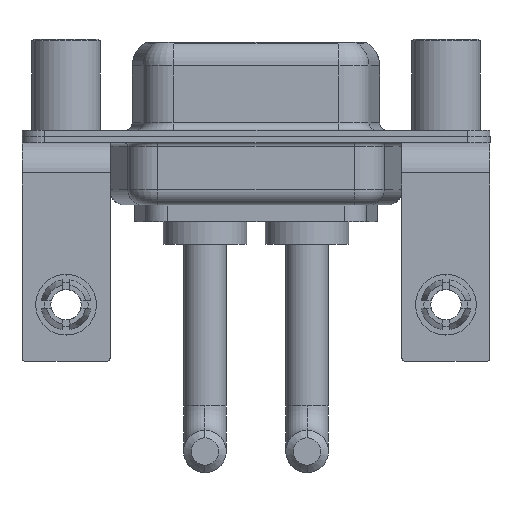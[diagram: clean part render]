
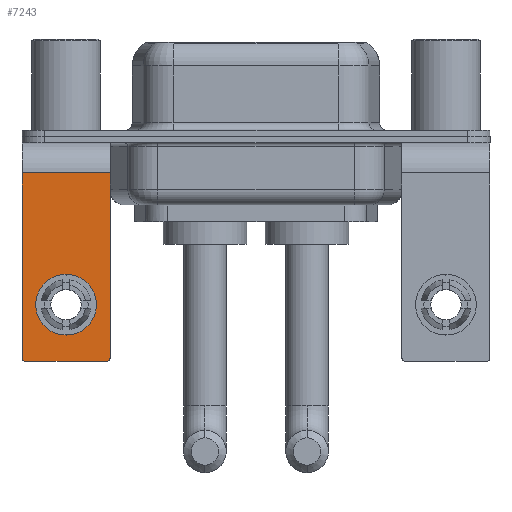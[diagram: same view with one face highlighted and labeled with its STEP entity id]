
A CAD part, front view. The second image highlights one B-rep face of the part: STEP entity #7243.
In plain terms, the highlighted planar face has unit normal (0, -1, 0).
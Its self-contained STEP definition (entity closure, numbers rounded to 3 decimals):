
#152 = CARTESIAN_POINT ( 'NONE',  ( 0., -6.25, -11.07 ) ) ;
#338 = CARTESIAN_POINT ( 'NONE',  ( -2.9, -6.25, -2.4 ) ) ;
#465 = EDGE_CURVE ( 'NONE', #13450, #3374, #11641, .T. ) ;
#503 = DIRECTION ( 'NONE',  ( -1., 0., 0. ) ) ;
#672 = ORIENTED_EDGE ( 'NONE', *, *, #465, .T. ) ;
#893 = ORIENTED_EDGE ( 'NONE', *, *, #1160, .T. ) ;
#938 = CIRCLE ( 'NONE', #4370, 0.25 ) ;
#1090 = VECTOR ( 'NONE', #503, 1000. ) ;
#1160 = EDGE_CURVE ( 'NONE', #13355, #6694, #11419, .T. ) ;
#1371 = EDGE_CURVE ( 'NONE', #15027, #4818, #5659, .T. ) ;
#1728 = CARTESIAN_POINT ( 'NONE',  ( -2.65, -6.25, -14.55 ) ) ;
#1903 = DIRECTION ( 'NONE',  ( -1., 0., 0. ) ) ;
#3374 = VERTEX_POINT ( 'NONE', #11373 ) ;
#3584 = CARTESIAN_POINT ( 'NONE',  ( -2.9, -6.25, -2.4 ) ) ;
#4300 = CARTESIAN_POINT ( 'NONE',  ( 2.9, -6.25, -14.8 ) ) ;
#4367 = EDGE_CURVE ( 'NONE', #13355, #13337, #13212, .T. ) ;
#4370 = AXIS2_PLACEMENT_3D ( 'NONE', #1728, #5377, #15424 ) ;
#4409 = CARTESIAN_POINT ( 'NONE',  ( 2.65, -6.25, -14.8 ) ) ;
#4795 = EDGE_CURVE ( 'NONE', #4818, #15027, #13446, .T. ) ;
#4818 = VERTEX_POINT ( 'NONE', #11869 ) ;
#4866 = FACE_BOUND ( 'NONE', #14062, .T. ) ;
#5190 = DIRECTION ( 'NONE',  ( 0., 1., 0. ) ) ;
#5377 = DIRECTION ( 'NONE',  ( 0., -1., 0. ) ) ;
#5379 = ORIENTED_EDGE ( 'NONE', *, *, #10912, .F. ) ;
#5548 = EDGE_CURVE ( 'NONE', #3374, #13337, #938, .T. ) ;
#5565 = EDGE_LOOP ( 'NONE', ( #672, #9443, #11120, #893, #5379, #10185 ) ) ;
#5645 = LINE ( 'NONE', #8033, #1090 ) ;
#5659 = CIRCLE ( 'NONE', #15913, 2. ) ;
#6426 = PLANE ( 'NONE',  #9418 ) ;
#6647 = LINE ( 'NONE', #6989, #9745 ) ;
#6694 = VERTEX_POINT ( 'NONE', #13332 ) ;
#6989 = CARTESIAN_POINT ( 'NONE',  ( 2.9, -6.25, -2.4 ) ) ;
#7184 = DIRECTION ( 'NONE',  ( 0., 0., 1. ) ) ;
#7243 = ADVANCED_FACE ( 'NONE', ( #4866, #11213 ), #6426, .F. ) ;
#7639 = DIRECTION ( 'NONE',  ( 0., 0., 1. ) ) ;
#7681 = VECTOR ( 'NONE', #8115, 1000. ) ;
#8033 = CARTESIAN_POINT ( 'NONE',  ( 2.9, -6.25, -2.4 ) ) ;
#8115 = DIRECTION ( 'NONE',  ( 0., 0., -1. ) ) ;
#8862 = CARTESIAN_POINT ( 'NONE',  ( 0., -6.25, -9.07 ) ) ;
#9036 = CARTESIAN_POINT ( 'NONE',  ( 0., -6.25, -11.07 ) ) ;
#9203 = CARTESIAN_POINT ( 'NONE',  ( 2.9, -6.25, -2.4 ) ) ;
#9418 = AXIS2_PLACEMENT_3D ( 'NONE', #13762, #14997, #11293 ) ;
#9443 = ORIENTED_EDGE ( 'NONE', *, *, #5548, .T. ) ;
#9745 = VECTOR ( 'NONE', #14384, 1000. ) ;
#9858 = AXIS2_PLACEMENT_3D ( 'NONE', #14589, #12122, #7184 ) ;
#10185 = ORIENTED_EDGE ( 'NONE', *, *, #13724, .T. ) ;
#10685 = CARTESIAN_POINT ( 'NONE',  ( -2.65, -6.25, -14.8 ) ) ;
#10912 = EDGE_CURVE ( 'NONE', #10919, #6694, #6647, .T. ) ;
#10919 = VERTEX_POINT ( 'NONE', #9203 ) ;
#11120 = ORIENTED_EDGE ( 'NONE', *, *, #4367, .F. ) ;
#11213 = FACE_OUTER_BOUND ( 'NONE', #5565, .T. ) ;
#11293 = DIRECTION ( 'NONE',  ( 0., 0., 1. ) ) ;
#11373 = CARTESIAN_POINT ( 'NONE',  ( -2.9, -6.25, -14.55 ) ) ;
#11419 = CIRCLE ( 'NONE', #9858, 0.25 ) ;
#11525 = ORIENTED_EDGE ( 'NONE', *, *, #4795, .T. ) ;
#11641 = LINE ( 'NONE', #338, #7681 ) ;
#11869 = CARTESIAN_POINT ( 'NONE',  ( 0., -6.25, -13.07 ) ) ;
#12122 = DIRECTION ( 'NONE',  ( 0., -1., 0. ) ) ;
#12899 = AXIS2_PLACEMENT_3D ( 'NONE', #152, #5190, #15244 ) ;
#12989 = ORIENTED_EDGE ( 'NONE', *, *, #1371, .T. ) ;
#13212 = LINE ( 'NONE', #4300, #14323 ) ;
#13332 = CARTESIAN_POINT ( 'NONE',  ( 2.9, -6.25, -14.55 ) ) ;
#13337 = VERTEX_POINT ( 'NONE', #10685 ) ;
#13355 = VERTEX_POINT ( 'NONE', #4409 ) ;
#13446 = CIRCLE ( 'NONE', #12899, 2. ) ;
#13450 = VERTEX_POINT ( 'NONE', #3584 ) ;
#13724 = EDGE_CURVE ( 'NONE', #10919, #13450, #5645, .T. ) ;
#13762 = CARTESIAN_POINT ( 'NONE',  ( 2.9, -6.25, -2.4 ) ) ;
#14055 = DIRECTION ( 'NONE',  ( 0., 1., 0. ) ) ;
#14062 = EDGE_LOOP ( 'NONE', ( #11525, #12989 ) ) ;
#14323 = VECTOR ( 'NONE', #1903, 1000. ) ;
#14384 = DIRECTION ( 'NONE',  ( 0., 0., -1. ) ) ;
#14589 = CARTESIAN_POINT ( 'NONE',  ( 2.65, -6.25, -14.55 ) ) ;
#14997 = DIRECTION ( 'NONE',  ( 0., 1., 0. ) ) ;
#15027 = VERTEX_POINT ( 'NONE', #8862 ) ;
#15244 = DIRECTION ( 'NONE',  ( 0., 0., 1. ) ) ;
#15424 = DIRECTION ( 'NONE',  ( 0., 0., 1. ) ) ;
#15913 = AXIS2_PLACEMENT_3D ( 'NONE', #9036, #14055, #7639 ) ;
